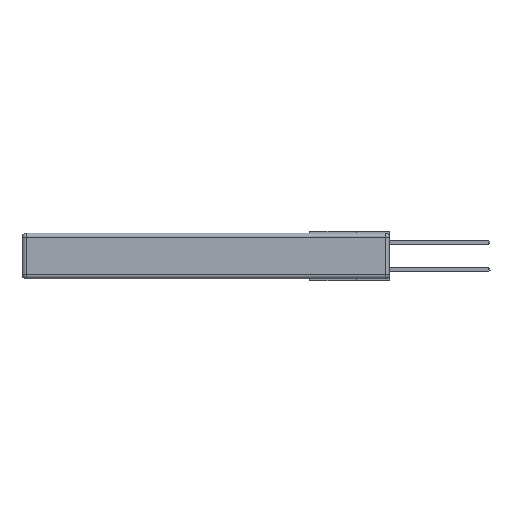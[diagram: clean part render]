
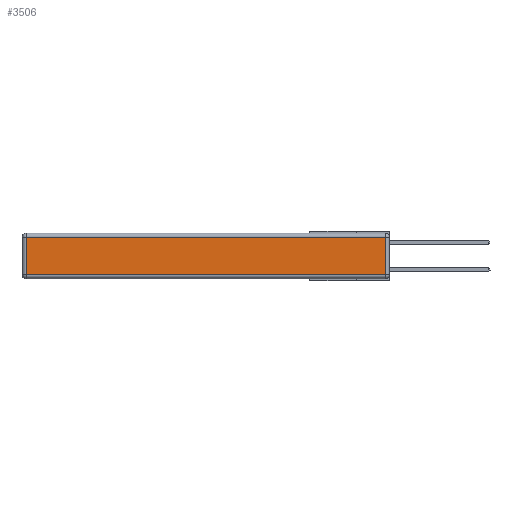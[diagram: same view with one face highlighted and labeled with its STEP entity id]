
A CAD part, left-side view. The second image highlights one B-rep face of the part: STEP entity #3506.
In plain terms, the highlighted planar face has unit normal (-1, 0, 0).
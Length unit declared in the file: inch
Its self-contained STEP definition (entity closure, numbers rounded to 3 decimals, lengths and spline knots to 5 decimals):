
#153 = CARTESIAN_POINT ( 'NONE',  ( 0., 0.03, -0.313 ) ) ;
#169 = VECTOR ( 'NONE', #6107, 39.37008 ) ;
#572 = CARTESIAN_POINT ( 'NONE',  ( 0., 0.03, -0.03 ) ) ;
#772 = VECTOR ( 'NONE', #8438, 39.37008 ) ;
#812 = DIRECTION ( 'NONE',  ( 0., 1., 0. ) ) ;
#1080 = CARTESIAN_POINT ( 'NONE',  ( 0., 0., -0.313 ) ) ;
#1156 = VECTOR ( 'NONE', #812, 39.37008 ) ;
#1786 = AXIS2_PLACEMENT_3D ( 'NONE', #10708, #3835, #8301 ) ;
#2332 = DIRECTION ( 'NONE',  ( 0., 0., 1. ) ) ;
#3506 = ADVANCED_FACE ( 'NONE', ( #10669 ), #3930, .T. ) ;
#3580 = EDGE_CURVE ( 'NONE', #13093, #10321, #9422, .T. ) ;
#3835 = DIRECTION ( 'NONE',  ( -1., 0., 0. ) ) ;
#3930 = PLANE ( 'NONE',  #1786 ) ;
#4572 = EDGE_CURVE ( 'NONE', #7118, #13093, #9165, .T. ) ;
#6107 = DIRECTION ( 'NONE',  ( 0., -1., 0. ) ) ;
#6401 = CARTESIAN_POINT ( 'NONE',  ( 0., 2.75, -0.03 ) ) ;
#6666 = ORIENTED_EDGE ( 'NONE', *, *, #9448, .T. ) ;
#7011 = VECTOR ( 'NONE', #2332, 39.37008 ) ;
#7118 = VERTEX_POINT ( 'NONE', #12150 ) ;
#7303 = EDGE_CURVE ( 'NONE', #10321, #10716, #7341, .T. ) ;
#7341 = LINE ( 'NONE', #9047, #7011 ) ;
#8301 = DIRECTION ( 'NONE',  ( 0., 0., 1. ) ) ;
#8438 = DIRECTION ( 'NONE',  ( 0., 0., -1. ) ) ;
#8531 = CARTESIAN_POINT ( 'NONE',  ( 0., 2.72, -0.343 ) ) ;
#9047 = CARTESIAN_POINT ( 'NONE',  ( 0., 0.03, -0.343 ) ) ;
#9165 = LINE ( 'NONE', #8531, #772 ) ;
#9422 = LINE ( 'NONE', #1080, #169 ) ;
#9448 = EDGE_CURVE ( 'NONE', #10716, #7118, #13379, .T. ) ;
#9520 = ORIENTED_EDGE ( 'NONE', *, *, #3580, .T. ) ;
#9991 = CARTESIAN_POINT ( 'NONE',  ( 0., 2.72, -0.313 ) ) ;
#10321 = VERTEX_POINT ( 'NONE', #153 ) ;
#10669 = FACE_OUTER_BOUND ( 'NONE', #11445, .T. ) ;
#10708 = CARTESIAN_POINT ( 'NONE',  ( 0., 0., -0.343 ) ) ;
#10716 = VERTEX_POINT ( 'NONE', #572 ) ;
#11399 = ORIENTED_EDGE ( 'NONE', *, *, #4572, .T. ) ;
#11445 = EDGE_LOOP ( 'NONE', ( #9520, #13822, #6666, #11399 ) ) ;
#12150 = CARTESIAN_POINT ( 'NONE',  ( 0., 2.72, -0.03 ) ) ;
#13093 = VERTEX_POINT ( 'NONE', #9991 ) ;
#13379 = LINE ( 'NONE', #6401, #1156 ) ;
#13822 = ORIENTED_EDGE ( 'NONE', *, *, #7303, .T. ) ;
